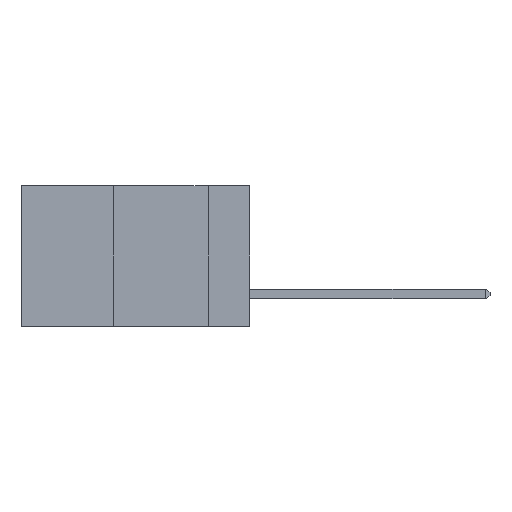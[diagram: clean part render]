
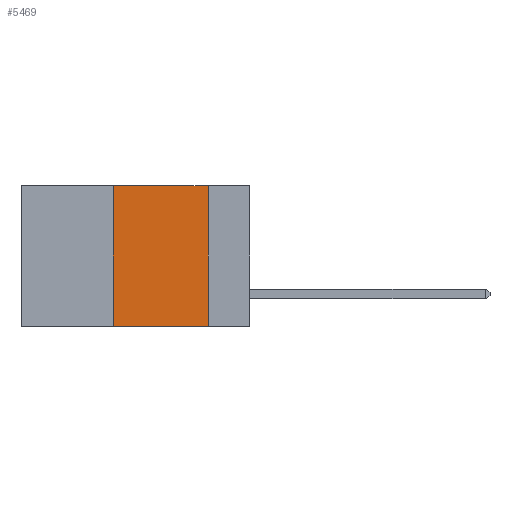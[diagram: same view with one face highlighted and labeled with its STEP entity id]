
A CAD part, left-side view. The second image highlights one B-rep face of the part: STEP entity #5469.
In plain terms, the highlighted planar face has unit normal (-1, 0, 0).
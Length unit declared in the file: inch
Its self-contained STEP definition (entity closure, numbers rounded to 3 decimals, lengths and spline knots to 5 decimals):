
#415 = EDGE_CURVE ( 'NONE', #4820, #16522, #9417, .T. ) ;
#601 = CARTESIAN_POINT ( 'NONE',  ( 0., 0.6, 0. ) ) ;
#829 = VECTOR ( 'NONE', #18582, 39.37008 ) ;
#1054 = VERTEX_POINT ( 'NONE', #13344 ) ;
#2353 = PLANE ( 'NONE',  #5940 ) ;
#4820 = VERTEX_POINT ( 'NONE', #15834 ) ;
#4865 = LINE ( 'NONE', #11211, #829 ) ;
#5230 = EDGE_CURVE ( 'NONE', #16522, #1054, #11761, .T. ) ;
#5260 = CARTESIAN_POINT ( 'NONE',  ( 0., 0.36, -0.37 ) ) ;
#5360 = EDGE_CURVE ( 'NONE', #11347, #1054, #4865, .T. ) ;
#5469 = ADVANCED_FACE ( 'NONE', ( #15015 ), #2353, .F. ) ;
#5940 = AXIS2_PLACEMENT_3D ( 'NONE', #12925, #6856, #17356 ) ;
#6856 = DIRECTION ( 'NONE',  ( 1., 0., 0. ) ) ;
#8170 = ORIENTED_EDGE ( 'NONE', *, *, #415, .F. ) ;
#8670 = ORIENTED_EDGE ( 'NONE', *, *, #14565, .F. ) ;
#9369 = CARTESIAN_POINT ( 'NONE',  ( 0., 0.11, 0. ) ) ;
#9417 = LINE ( 'NONE', #601, #12966 ) ;
#9478 = DIRECTION ( 'NONE',  ( 0., -1., 0. ) ) ;
#10614 = DIRECTION ( 'NONE',  ( 0., 0., 1. ) ) ;
#10876 = DIRECTION ( 'NONE',  ( 0., 0., -1. ) ) ;
#11211 = CARTESIAN_POINT ( 'NONE',  ( 0., 0.6, -0.37 ) ) ;
#11347 = VERTEX_POINT ( 'NONE', #5260 ) ;
#11761 = LINE ( 'NONE', #9369, #19129 ) ;
#12029 = VECTOR ( 'NONE', #10614, 39.37008 ) ;
#12821 = EDGE_LOOP ( 'NONE', ( #14790, #8170, #8670, #18250 ) ) ;
#12925 = CARTESIAN_POINT ( 'NONE',  ( 0., 0.6, 0. ) ) ;
#12966 = VECTOR ( 'NONE', #9478, 39.37008 ) ;
#13344 = CARTESIAN_POINT ( 'NONE',  ( 0., 0.11, -0.37 ) ) ;
#14565 = EDGE_CURVE ( 'NONE', #11347, #4820, #15948, .T. ) ;
#14790 = ORIENTED_EDGE ( 'NONE', *, *, #5230, .F. ) ;
#15015 = FACE_OUTER_BOUND ( 'NONE', #12821, .T. ) ;
#15072 = CARTESIAN_POINT ( 'NONE',  ( 0., 0.36, 0. ) ) ;
#15834 = CARTESIAN_POINT ( 'NONE',  ( 0., 0.36, 0. ) ) ;
#15939 = CARTESIAN_POINT ( 'NONE',  ( 0., 0.11, 0. ) ) ;
#15948 = LINE ( 'NONE', #15072, #12029 ) ;
#16522 = VERTEX_POINT ( 'NONE', #15939 ) ;
#17356 = DIRECTION ( 'NONE',  ( 0., 0., -1. ) ) ;
#18250 = ORIENTED_EDGE ( 'NONE', *, *, #5360, .T. ) ;
#18582 = DIRECTION ( 'NONE',  ( 0., -1., 0. ) ) ;
#19129 = VECTOR ( 'NONE', #10876, 39.37008 ) ;
